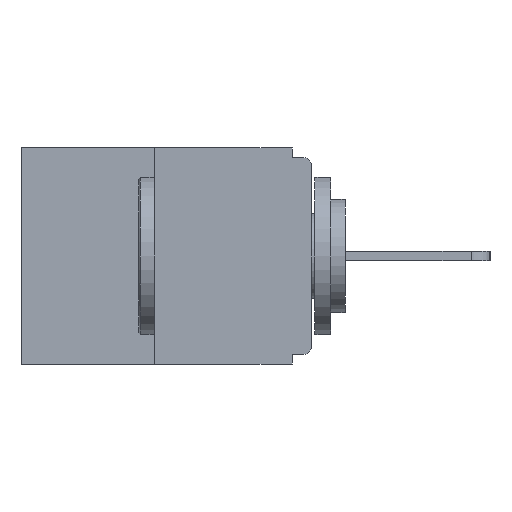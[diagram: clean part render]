
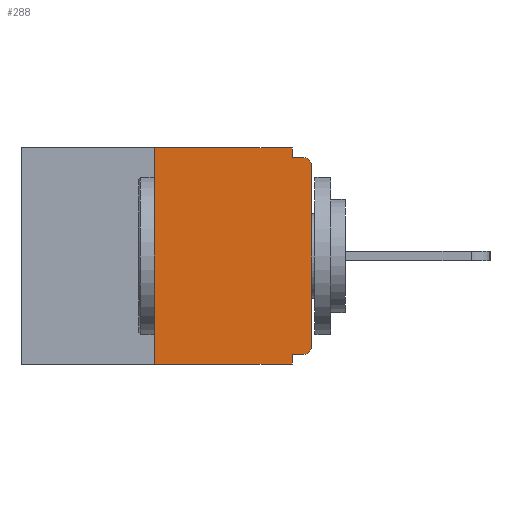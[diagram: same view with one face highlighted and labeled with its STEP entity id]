
A CAD part, left-side view. The second image highlights one B-rep face of the part: STEP entity #288.
In plain terms, the highlighted planar face has unit normal (-1, 0, 0).
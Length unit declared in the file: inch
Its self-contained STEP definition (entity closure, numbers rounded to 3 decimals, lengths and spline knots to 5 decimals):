
#50 = DIRECTION ( 'NONE',  ( -1., 0., 0. ) ) ;
#151 = CARTESIAN_POINT ( 'NONE',  ( 0., 0.46, 0. ) ) ;
#288 = ADVANCED_FACE ( 'NONE', ( #14228 ), #9168, .F. ) ;
#547 = VECTOR ( 'NONE', #2608, 39.37008 ) ;
#752 = EDGE_CURVE ( 'NONE', #8198, #11574, #7302, .T. ) ;
#1136 = CARTESIAN_POINT ( 'NONE',  ( 0., 0., -0.015 ) ) ;
#1272 = DIRECTION ( 'NONE',  ( 0., 0., -1. ) ) ;
#1522 = EDGE_CURVE ( 'NONE', #14473, #6280, #9344, .T. ) ;
#1600 = LINE ( 'NONE', #1136, #13962 ) ;
#1961 = DIRECTION ( 'NONE',  ( -1., 0., 0. ) ) ;
#2384 = EDGE_CURVE ( 'NONE', #2467, #9364, #10455, .T. ) ;
#2467 = VERTEX_POINT ( 'NONE', #4330 ) ;
#2519 = VECTOR ( 'NONE', #5685, 39.37008 ) ;
#2536 = ORIENTED_EDGE ( 'NONE', *, *, #6967, .F. ) ;
#2608 = DIRECTION ( 'NONE',  ( 0., 0., 1. ) ) ;
#2910 = ORIENTED_EDGE ( 'NONE', *, *, #752, .T. ) ;
#2948 = VECTOR ( 'NONE', #14843, 39.37008 ) ;
#2992 = DIRECTION ( 'NONE',  ( 0., 0., -1. ) ) ;
#3142 = DIRECTION ( 'NONE',  ( 1., 0., 0. ) ) ;
#3227 = DIRECTION ( 'NONE',  ( 0., 0., -1. ) ) ;
#3439 = EDGE_CURVE ( 'NONE', #9364, #9308, #1600, .T. ) ;
#3680 = CARTESIAN_POINT ( 'NONE',  ( 0., 0.015, -0.313 ) ) ;
#3708 = ORIENTED_EDGE ( 'NONE', *, *, #1522, .F. ) ;
#4165 = ORIENTED_EDGE ( 'NONE', *, *, #15123, .T. ) ;
#4215 = CARTESIAN_POINT ( 'NONE',  ( 0., 0.25, 0. ) ) ;
#4330 = CARTESIAN_POINT ( 'NONE',  ( 0., 0.031, 0. ) ) ;
#4420 = DIRECTION ( 'NONE',  ( 0., -1., 0. ) ) ;
#4499 = CARTESIAN_POINT ( 'NONE',  ( 0., 0., -0.313 ) ) ;
#4645 = VECTOR ( 'NONE', #3227, 39.37008 ) ;
#4646 = CARTESIAN_POINT ( 'NONE',  ( 0., 0.015, -0.03 ) ) ;
#4982 = ORIENTED_EDGE ( 'NONE', *, *, #2384, .F. ) ;
#5032 = EDGE_LOOP ( 'NONE', ( #2536, #14527, #4165, #3708, #12597, #8225, #2910, #11734, #11202, #4982 ) ) ;
#5439 = EDGE_CURVE ( 'NONE', #11574, #9308, #13336, .T. ) ;
#5475 = AXIS2_PLACEMENT_3D ( 'NONE', #3680, #50, #1272 ) ;
#5552 = CARTESIAN_POINT ( 'NONE',  ( 0., 0.46, 0. ) ) ;
#5591 = CARTESIAN_POINT ( 'NONE',  ( 0., 0.015, -0.328 ) ) ;
#5685 = DIRECTION ( 'NONE',  ( 0., -1., 0. ) ) ;
#5741 = CARTESIAN_POINT ( 'NONE',  ( 0., 0.031, -0.343 ) ) ;
#6124 = LINE ( 'NONE', #12550, #2948 ) ;
#6280 = VERTEX_POINT ( 'NONE', #5741 ) ;
#6967 = EDGE_CURVE ( 'NONE', #10488, #2467, #13942, .T. ) ;
#7302 = LINE ( 'NONE', #7349, #547 ) ;
#7322 = DIRECTION ( 'NONE',  ( 0., -1., 0. ) ) ;
#7349 = CARTESIAN_POINT ( 'NONE',  ( 0., 0., 0. ) ) ;
#8122 = LINE ( 'NONE', #4215, #9647 ) ;
#8198 = VERTEX_POINT ( 'NONE', #4499 ) ;
#8225 = ORIENTED_EDGE ( 'NONE', *, *, #14336, .T. ) ;
#8499 = CARTESIAN_POINT ( 'NONE',  ( 0., 0.25, -0.343 ) ) ;
#8801 = DIRECTION ( 'NONE',  ( 0., 0., -1. ) ) ;
#8963 = CARTESIAN_POINT ( 'NONE',  ( 0., 0.031, 0. ) ) ;
#9148 = DIRECTION ( 'NONE',  ( 0., 0., -1. ) ) ;
#9168 = PLANE ( 'NONE',  #15351 ) ;
#9308 = VERTEX_POINT ( 'NONE', #14994 ) ;
#9344 = LINE ( 'NONE', #12744, #4645 ) ;
#9364 = VERTEX_POINT ( 'NONE', #15263 ) ;
#9647 = VECTOR ( 'NONE', #12582, 39.37008 ) ;
#9779 = VERTEX_POINT ( 'NONE', #8499 ) ;
#10267 = VECTOR ( 'NONE', #8801, 39.37008 ) ;
#10455 = LINE ( 'NONE', #8963, #10267 ) ;
#10488 = VERTEX_POINT ( 'NONE', #12233 ) ;
#11202 = ORIENTED_EDGE ( 'NONE', *, *, #3439, .F. ) ;
#11461 = CARTESIAN_POINT ( 'NONE',  ( 0., 0.031, -0.328 ) ) ;
#11574 = VERTEX_POINT ( 'NONE', #12969 ) ;
#11644 = CARTESIAN_POINT ( 'NONE',  ( 0., 0.46, -0.343 ) ) ;
#11734 = ORIENTED_EDGE ( 'NONE', *, *, #5439, .T. ) ;
#12233 = CARTESIAN_POINT ( 'NONE',  ( 0., 0.25, 0. ) ) ;
#12457 = CIRCLE ( 'NONE', #5475, 0.015 ) ;
#12550 = CARTESIAN_POINT ( 'NONE',  ( 0., 0., -0.328 ) ) ;
#12582 = DIRECTION ( 'NONE',  ( 0., 0., 1. ) ) ;
#12597 = ORIENTED_EDGE ( 'NONE', *, *, #13655, .F. ) ;
#12744 = CARTESIAN_POINT ( 'NONE',  ( 0., 0.031, -0.343 ) ) ;
#12969 = CARTESIAN_POINT ( 'NONE',  ( 0., 0., -0.03 ) ) ;
#13198 = VECTOR ( 'NONE', #7322, 39.37008 ) ;
#13336 = CIRCLE ( 'NONE', #14425, 0.015 ) ;
#13547 = LINE ( 'NONE', #11644, #2519 ) ;
#13655 = EDGE_CURVE ( 'NONE', #14217, #14473, #6124, .T. ) ;
#13942 = LINE ( 'NONE', #151, #13198 ) ;
#13962 = VECTOR ( 'NONE', #4420, 39.37008 ) ;
#14217 = VERTEX_POINT ( 'NONE', #5591 ) ;
#14228 = FACE_OUTER_BOUND ( 'NONE', #5032, .T. ) ;
#14336 = EDGE_CURVE ( 'NONE', #14217, #8198, #12457, .T. ) ;
#14425 = AXIS2_PLACEMENT_3D ( 'NONE', #4646, #1961, #9148 ) ;
#14473 = VERTEX_POINT ( 'NONE', #11461 ) ;
#14527 = ORIENTED_EDGE ( 'NONE', *, *, #15011, .F. ) ;
#14843 = DIRECTION ( 'NONE',  ( 0., 1., 0. ) ) ;
#14994 = CARTESIAN_POINT ( 'NONE',  ( 0., 0.015, -0.015 ) ) ;
#15011 = EDGE_CURVE ( 'NONE', #9779, #10488, #8122, .T. ) ;
#15123 = EDGE_CURVE ( 'NONE', #9779, #6280, #13547, .T. ) ;
#15263 = CARTESIAN_POINT ( 'NONE',  ( 0., 0.031, -0.015 ) ) ;
#15351 = AXIS2_PLACEMENT_3D ( 'NONE', #5552, #3142, #2992 ) ;
